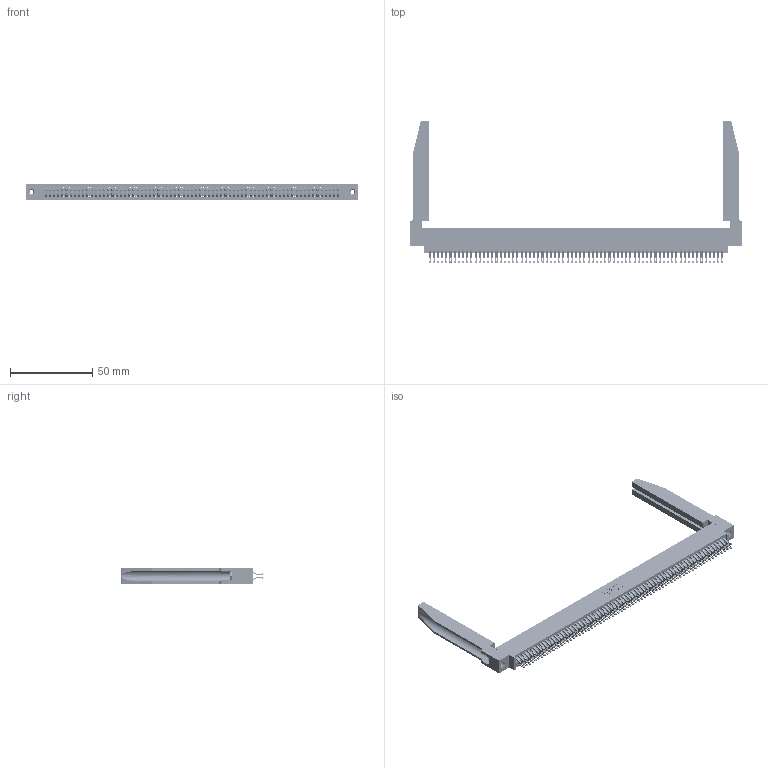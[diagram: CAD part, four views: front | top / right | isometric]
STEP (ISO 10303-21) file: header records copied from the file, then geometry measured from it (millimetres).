
FILE_DESCRIPTION (( 'STEP AP203' ), '1' );
FILE_NAME ('345-142-555-878.STEP', '2019-11-09T04:34:46', ( '' ), ( '' ), 'SwSTEP 2.0', 'SolidWorks 2016', '' );
FILE_SCHEMA (( 'CONFIG_CONTROL_DESIGN' ));
Length unit declared in the file: inch
Products named in the file (5): 345 Part_0.170 Offset - 0.156 Dia-TH; 345-250-001_345-250-001-102; 345-142-555-878; 345-292-001_555 Tail; 345-220-078_345-220-078
Assembly tree (147 placements, depth 2):
  345-142-555-878
    345 Part_0.170 Offset - 0.156 Dia-TH
    345-292-001_555 Tail  x142
    345-250-001_345-250-001-102  x2
    345-220-078_345-220-078  x2
Bounding box: 201.57 x 86.41 x 9.4 mm (x, y, z)
Volume: 27919.3 mm3; surface area: 38759.5 mm2
Topology: 147 solids, 147 shells, 8316 faces, 26095 edges, 17386 vertices
Faces by surface type: plane 4628, cylinder 3636, bspline 36, cone 12, torus 4
Entity records: 57002 total; most frequent: CARTESIAN_POINT 10481, ORIENTED_EDGE 9282, DIRECTION 8167, EDGE_CURVE 4641, VECTOR 4111, LINE 4111, VERTEX_POINT 3088, AXIS2_PLACEMENT_3D 2028
